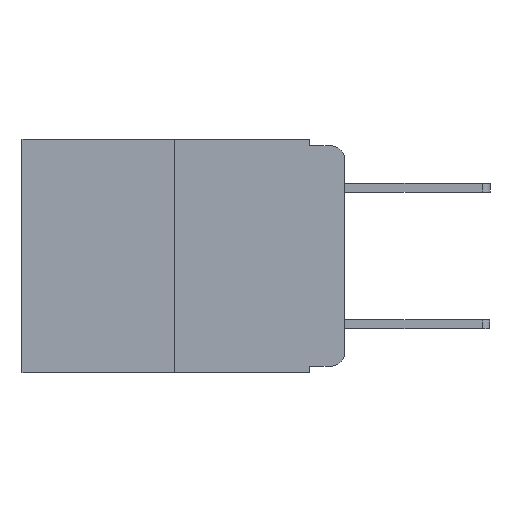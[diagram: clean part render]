
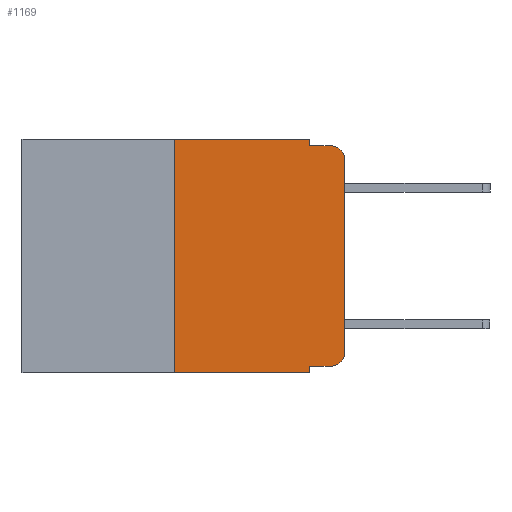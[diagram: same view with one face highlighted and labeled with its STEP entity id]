
A CAD part, left-side view. The second image highlights one B-rep face of the part: STEP entity #1169.
In plain terms, the highlighted planar face has unit normal (-1, 0, 0).
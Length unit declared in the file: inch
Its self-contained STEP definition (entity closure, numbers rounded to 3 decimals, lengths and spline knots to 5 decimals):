
#29 = CARTESIAN_POINT ( 'NONE',  ( 0., 0.473, 0. ) ) ;
#117 = ORIENTED_EDGE ( 'NONE', *, *, #2533, .F. ) ;
#219 = CARTESIAN_POINT ( 'NONE',  ( 0., 0.25, 0. ) ) ;
#242 = CARTESIAN_POINT ( 'NONE',  ( 0., 0.02, -0.333 ) ) ;
#547 = ORIENTED_EDGE ( 'NONE', *, *, #2300, .T. ) ;
#659 = CARTESIAN_POINT ( 'NONE',  ( 0., 0.051, 0. ) ) ;
#710 = DIRECTION ( 'NONE',  ( 0., 0., -1. ) ) ;
#738 = DIRECTION ( 'NONE',  ( -1., 0., 0. ) ) ;
#755 = CARTESIAN_POINT ( 'NONE',  ( 0., 0.02, -0.03 ) ) ;
#848 = PLANE ( 'NONE',  #8781 ) ;
#1127 = DIRECTION ( 'NONE',  ( 0., -1., 0. ) ) ;
#1169 = ADVANCED_FACE ( 'NONE', ( #11954 ), #848, .F. ) ;
#1335 = DIRECTION ( 'NONE',  ( 0., 0., -1. ) ) ;
#1671 = EDGE_CURVE ( 'NONE', #5685, #3708, #12670, .T. ) ;
#1845 = CARTESIAN_POINT ( 'NONE',  ( 0., 0.051, -0.333 ) ) ;
#2300 = EDGE_CURVE ( 'NONE', #9811, #11358, #6026, .T. ) ;
#2447 = EDGE_CURVE ( 'NONE', #11358, #11850, #6945, .T. ) ;
#2473 = EDGE_CURVE ( 'NONE', #2991, #11850, #6572, .T. ) ;
#2507 = VECTOR ( 'NONE', #4156, 39.37008 ) ;
#2533 = EDGE_CURVE ( 'NONE', #8036, #2991, #5838, .T. ) ;
#2582 = EDGE_CURVE ( 'NONE', #5685, #7713, #8630, .T. ) ;
#2767 = EDGE_CURVE ( 'NONE', #11488, #3708, #6748, .T. ) ;
#2790 = EDGE_CURVE ( 'NONE', #11488, #10165, #9507, .T. ) ;
#2814 = EDGE_CURVE ( 'NONE', #10165, #9811, #15304, .T. ) ;
#2968 = CARTESIAN_POINT ( 'NONE',  ( 0., 0.473, 0. ) ) ;
#2983 = CARTESIAN_POINT ( 'NONE',  ( 0., 0., -0.03 ) ) ;
#2991 = VERTEX_POINT ( 'NONE', #10370 ) ;
#3551 = ORIENTED_EDGE ( 'NONE', *, *, #2767, .F. ) ;
#3708 = VERTEX_POINT ( 'NONE', #10971 ) ;
#4113 = ORIENTED_EDGE ( 'NONE', *, *, #2447, .T. ) ;
#4156 = DIRECTION ( 'NONE',  ( 0., -1., 0. ) ) ;
#4630 = VECTOR ( 'NONE', #13484, 39.37008 ) ;
#5400 = DIRECTION ( 'NONE',  ( 0., 0., -1. ) ) ;
#5685 = VERTEX_POINT ( 'NONE', #10521 ) ;
#5834 = CARTESIAN_POINT ( 'NONE',  ( 0., 0., -0.313 ) ) ;
#5838 = LINE ( 'NONE', #12711, #11625 ) ;
#6026 = LINE ( 'NONE', #6398, #14667 ) ;
#6380 = VECTOR ( 'NONE', #1127, 39.37008 ) ;
#6398 = CARTESIAN_POINT ( 'NONE',  ( 0., 0., 0. ) ) ;
#6525 = EDGE_LOOP ( 'NONE', ( #547, #4113, #10038, #117, #10250, #14586, #11714, #3551, #11383, #6563 ) ) ;
#6563 = ORIENTED_EDGE ( 'NONE', *, *, #2814, .T. ) ;
#6572 = LINE ( 'NONE', #6828, #12315 ) ;
#6748 = LINE ( 'NONE', #659, #12466 ) ;
#6828 = CARTESIAN_POINT ( 'NONE',  ( 0., 0.051, -0.01 ) ) ;
#6945 = CIRCLE ( 'NONE', #8902, 0.02 ) ;
#7713 = VERTEX_POINT ( 'NONE', #219 ) ;
#8036 = VERTEX_POINT ( 'NONE', #11825 ) ;
#8551 = CARTESIAN_POINT ( 'NONE',  ( 0., 0.051, -0.333 ) ) ;
#8630 = LINE ( 'NONE', #12770, #4630 ) ;
#8781 = AXIS2_PLACEMENT_3D ( 'NONE', #2968, #10755, #5400 ) ;
#8902 = AXIS2_PLACEMENT_3D ( 'NONE', #755, #738, #710 ) ;
#9455 = LINE ( 'NONE', #29, #2507 ) ;
#9507 = LINE ( 'NONE', #8551, #6380 ) ;
#9711 = VECTOR ( 'NONE', #12156, 39.37008 ) ;
#9731 = CARTESIAN_POINT ( 'NONE',  ( 0., 0.02, -0.01 ) ) ;
#9811 = VERTEX_POINT ( 'NONE', #5834 ) ;
#10038 = ORIENTED_EDGE ( 'NONE', *, *, #2473, .F. ) ;
#10097 = DIRECTION ( 'NONE',  ( 0., 0., 1. ) ) ;
#10165 = VERTEX_POINT ( 'NONE', #242 ) ;
#10250 = ORIENTED_EDGE ( 'NONE', *, *, #12441, .F. ) ;
#10370 = CARTESIAN_POINT ( 'NONE',  ( 0., 0.051, -0.01 ) ) ;
#10521 = CARTESIAN_POINT ( 'NONE',  ( 0., 0.25, -0.343 ) ) ;
#10755 = DIRECTION ( 'NONE',  ( 1., 0., 0. ) ) ;
#10971 = CARTESIAN_POINT ( 'NONE',  ( 0., 0.051, -0.343 ) ) ;
#11358 = VERTEX_POINT ( 'NONE', #2983 ) ;
#11383 = ORIENTED_EDGE ( 'NONE', *, *, #2790, .T. ) ;
#11488 = VERTEX_POINT ( 'NONE', #1845 ) ;
#11625 = VECTOR ( 'NONE', #1335, 39.37008 ) ;
#11714 = ORIENTED_EDGE ( 'NONE', *, *, #1671, .T. ) ;
#11825 = CARTESIAN_POINT ( 'NONE',  ( 0., 0.051, 0. ) ) ;
#11850 = VERTEX_POINT ( 'NONE', #9731 ) ;
#11954 = FACE_OUTER_BOUND ( 'NONE', #6525, .T. ) ;
#12156 = DIRECTION ( 'NONE',  ( 0., -1., 0. ) ) ;
#12315 = VECTOR ( 'NONE', #12897, 39.37008 ) ;
#12425 = DIRECTION ( 'NONE',  ( 0., 0., -1. ) ) ;
#12441 = EDGE_CURVE ( 'NONE', #7713, #8036, #9455, .T. ) ;
#12466 = VECTOR ( 'NONE', #14344, 39.37008 ) ;
#12670 = LINE ( 'NONE', #14846, #9711 ) ;
#12711 = CARTESIAN_POINT ( 'NONE',  ( 0., 0.051, 0. ) ) ;
#12770 = CARTESIAN_POINT ( 'NONE',  ( 0., 0.25, 0. ) ) ;
#12785 = DIRECTION ( 'NONE',  ( -1., 0., 0. ) ) ;
#12897 = DIRECTION ( 'NONE',  ( 0., -1., 0. ) ) ;
#13484 = DIRECTION ( 'NONE',  ( 0., 0., 1. ) ) ;
#14228 = CARTESIAN_POINT ( 'NONE',  ( 0., 0.02, -0.313 ) ) ;
#14344 = DIRECTION ( 'NONE',  ( 0., 0., -1. ) ) ;
#14586 = ORIENTED_EDGE ( 'NONE', *, *, #2582, .F. ) ;
#14667 = VECTOR ( 'NONE', #10097, 39.37008 ) ;
#14846 = CARTESIAN_POINT ( 'NONE',  ( 0., 0.473, -0.343 ) ) ;
#15227 = AXIS2_PLACEMENT_3D ( 'NONE', #14228, #12785, #12425 ) ;
#15304 = CIRCLE ( 'NONE', #15227, 0.02 ) ;
